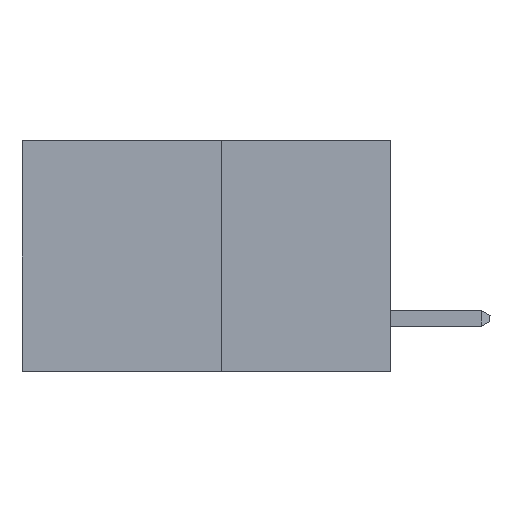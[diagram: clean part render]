
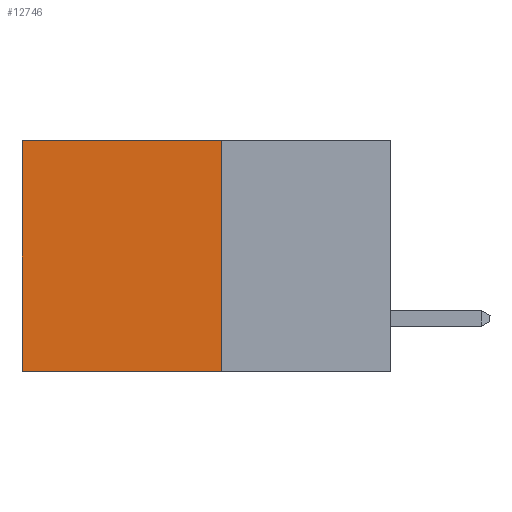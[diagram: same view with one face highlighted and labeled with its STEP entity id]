
A CAD part, left-side view. The second image highlights one B-rep face of the part: STEP entity #12746.
In plain terms, the highlighted planar face has unit normal (-1, 0, 0).
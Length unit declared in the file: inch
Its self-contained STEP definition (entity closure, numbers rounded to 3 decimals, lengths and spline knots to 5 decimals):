
#935 = VERTEX_POINT ( 'NONE', #8316 ) ;
#1182 = EDGE_CURVE ( 'NONE', #13745, #935, #6642, .T. ) ;
#1368 = CARTESIAN_POINT ( 'NONE',  ( 0.277, 0.27, -0.37 ) ) ;
#2880 = VECTOR ( 'NONE', #6490, 39.37008 ) ;
#3195 = EDGE_CURVE ( 'NONE', #7986, #13745, #13018, .T. ) ;
#4022 = CARTESIAN_POINT ( 'NONE',  ( 0.277, 0.59, 0. ) ) ;
#4406 = DIRECTION ( 'NONE',  ( 0., 1., 0. ) ) ;
#4664 = VERTEX_POINT ( 'NONE', #4022 ) ;
#5163 = LINE ( 'NONE', #8172, #13759 ) ;
#6334 = ORIENTED_EDGE ( 'NONE', *, *, #1182, .F. ) ;
#6490 = DIRECTION ( 'NONE',  ( 0., 1., 0. ) ) ;
#6642 = LINE ( 'NONE', #10139, #2880 ) ;
#7121 = CARTESIAN_POINT ( 'NONE',  ( 0.277, 0.27, -0.37 ) ) ;
#7986 = VERTEX_POINT ( 'NONE', #10273 ) ;
#8053 = DIRECTION ( 'NONE',  ( 0., 0., -1. ) ) ;
#8172 = CARTESIAN_POINT ( 'NONE',  ( 0.277, 0.27, 0. ) ) ;
#8316 = CARTESIAN_POINT ( 'NONE',  ( 0.277, 0.59, -0.37 ) ) ;
#8697 = ORIENTED_EDGE ( 'NONE', *, *, #8716, .T. ) ;
#8716 = EDGE_CURVE ( 'NONE', #7986, #4664, #5163, .T. ) ;
#9057 = VECTOR ( 'NONE', #8053, 39.37008 ) ;
#9184 = EDGE_CURVE ( 'NONE', #4664, #935, #12668, .T. ) ;
#9700 = PLANE ( 'NONE',  #11223 ) ;
#9991 = DIRECTION ( 'NONE',  ( 0., 0., -1. ) ) ;
#10089 = EDGE_LOOP ( 'NONE', ( #10457, #6334, #11957, #8697 ) ) ;
#10139 = CARTESIAN_POINT ( 'NONE',  ( 0.277, 0.27, -0.37 ) ) ;
#10273 = CARTESIAN_POINT ( 'NONE',  ( 0.277, 0.27, 0. ) ) ;
#10457 = ORIENTED_EDGE ( 'NONE', *, *, #9184, .T. ) ;
#11156 = CARTESIAN_POINT ( 'NONE',  ( 0.277, 0.27, -0.37 ) ) ;
#11223 = AXIS2_PLACEMENT_3D ( 'NONE', #7121, #14353, #12100 ) ;
#11740 = CARTESIAN_POINT ( 'NONE',  ( 0.277, 0.59, -0.37 ) ) ;
#11957 = ORIENTED_EDGE ( 'NONE', *, *, #3195, .F. ) ;
#12100 = DIRECTION ( 'NONE',  ( 0., 0., -1. ) ) ;
#12668 = LINE ( 'NONE', #11740, #9057 ) ;
#12746 = ADVANCED_FACE ( 'NONE', ( #14604 ), #9700, .F. ) ;
#13018 = LINE ( 'NONE', #11156, #15337 ) ;
#13745 = VERTEX_POINT ( 'NONE', #1368 ) ;
#13759 = VECTOR ( 'NONE', #4406, 39.37008 ) ;
#14353 = DIRECTION ( 'NONE',  ( 1., 0., 0. ) ) ;
#14604 = FACE_OUTER_BOUND ( 'NONE', #10089, .T. ) ;
#15337 = VECTOR ( 'NONE', #9991, 39.37008 ) ;
